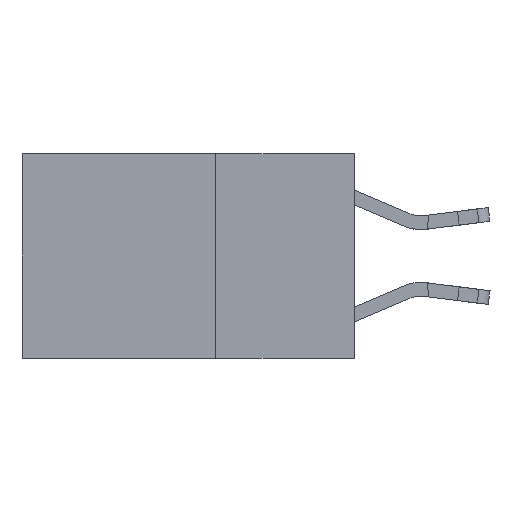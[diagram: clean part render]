
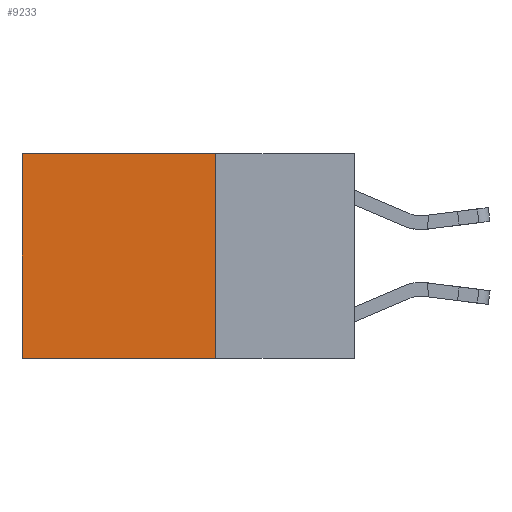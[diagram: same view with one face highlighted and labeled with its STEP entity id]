
A CAD part, left-side view. The second image highlights one B-rep face of the part: STEP entity #9233.
In plain terms, the highlighted planar face has unit normal (-1, 0, 0).
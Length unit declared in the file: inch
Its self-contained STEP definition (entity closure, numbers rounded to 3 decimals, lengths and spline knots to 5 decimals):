
#219 = ORIENTED_EDGE ( 'NONE', *, *, #5165, .F. ) ;
#1131 = EDGE_CURVE ( 'NONE', #11965, #4047, #7429, .T. ) ;
#1993 = DIRECTION ( 'NONE',  ( 0., 0., -1. ) ) ;
#2525 = DIRECTION ( 'NONE',  ( 0., 1., 0. ) ) ;
#2735 = CARTESIAN_POINT ( 'NONE',  ( 0.2625, 0.6, 0. ) ) ;
#3419 = DIRECTION ( 'NONE',  ( 0., 1., 0. ) ) ;
#3522 = LINE ( 'NONE', #7146, #3981 ) ;
#3948 = VERTEX_POINT ( 'NONE', #13439 ) ;
#3981 = VECTOR ( 'NONE', #2525, 39.37008 ) ;
#4015 = LINE ( 'NONE', #5124, #18183 ) ;
#4047 = VERTEX_POINT ( 'NONE', #18203 ) ;
#5124 = CARTESIAN_POINT ( 'NONE',  ( 0.2625, 0.25, 0. ) ) ;
#5165 = EDGE_CURVE ( 'NONE', #11965, #3948, #4015, .T. ) ;
#5909 = EDGE_CURVE ( 'NONE', #3948, #18629, #3522, .T. ) ;
#6303 = DIRECTION ( 'NONE',  ( 1., 0., 0. ) ) ;
#7146 = CARTESIAN_POINT ( 'NONE',  ( 0.2625, 0.25, -0.37 ) ) ;
#7429 = LINE ( 'NONE', #13664, #17223 ) ;
#9233 = ADVANCED_FACE ( 'NONE', ( #17613 ), #12388, .F. ) ;
#10215 = ORIENTED_EDGE ( 'NONE', *, *, #1131, .T. ) ;
#11833 = VECTOR ( 'NONE', #14380, 39.37008 ) ;
#11965 = VERTEX_POINT ( 'NONE', #12661 ) ;
#12388 = PLANE ( 'NONE',  #13838 ) ;
#12661 = CARTESIAN_POINT ( 'NONE',  ( 0.2625, 0.25, 0. ) ) ;
#12695 = ORIENTED_EDGE ( 'NONE', *, *, #16796, .T. ) ;
#13439 = CARTESIAN_POINT ( 'NONE',  ( 0.2625, 0.25, -0.37 ) ) ;
#13530 = CARTESIAN_POINT ( 'NONE',  ( 0.2625, 0.25, 0. ) ) ;
#13664 = CARTESIAN_POINT ( 'NONE',  ( 0.2625, 0.25, 0. ) ) ;
#13838 = AXIS2_PLACEMENT_3D ( 'NONE', #13530, #6303, #1993 ) ;
#14380 = DIRECTION ( 'NONE',  ( 0., 0., -1. ) ) ;
#16737 = DIRECTION ( 'NONE',  ( 0., 0., -1. ) ) ;
#16796 = EDGE_CURVE ( 'NONE', #4047, #18629, #18735, .T. ) ;
#17223 = VECTOR ( 'NONE', #3419, 39.37008 ) ;
#17573 = ORIENTED_EDGE ( 'NONE', *, *, #5909, .F. ) ;
#17613 = FACE_OUTER_BOUND ( 'NONE', #17978, .T. ) ;
#17978 = EDGE_LOOP ( 'NONE', ( #12695, #17573, #219, #10215 ) ) ;
#18174 = CARTESIAN_POINT ( 'NONE',  ( 0.2625, 0.6, -0.37 ) ) ;
#18183 = VECTOR ( 'NONE', #16737, 39.37008 ) ;
#18203 = CARTESIAN_POINT ( 'NONE',  ( 0.2625, 0.6, 0. ) ) ;
#18629 = VERTEX_POINT ( 'NONE', #18174 ) ;
#18735 = LINE ( 'NONE', #2735, #11833 ) ;
